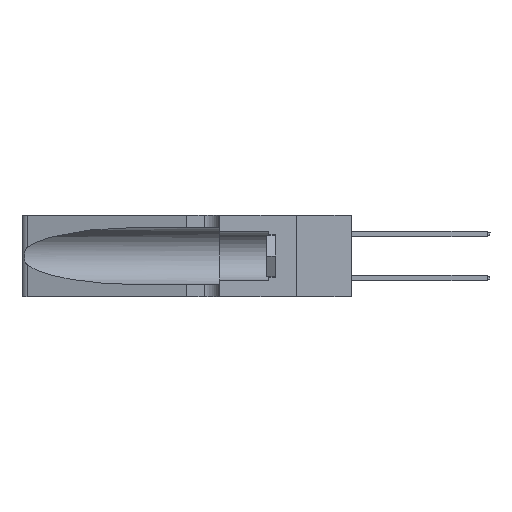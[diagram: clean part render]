
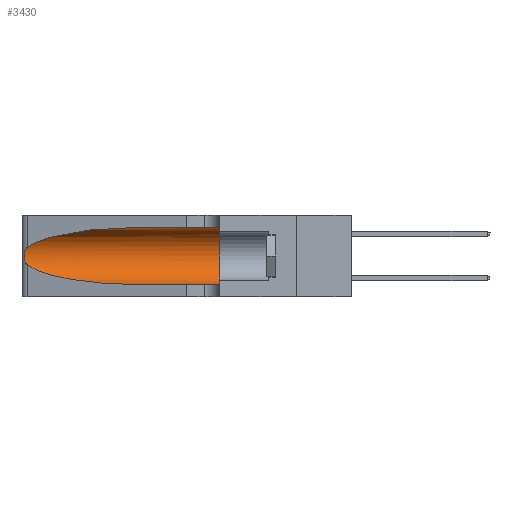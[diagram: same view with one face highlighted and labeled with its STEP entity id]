
A CAD part, left-side view. The second image highlights one B-rep face of the part: STEP entity #3430.
In plain terms, the highlighted cylindrical face has radius 3.308 mm (diameter 6.617 mm), a partial arc.
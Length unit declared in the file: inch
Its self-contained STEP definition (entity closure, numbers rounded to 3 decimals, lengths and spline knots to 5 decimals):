
#22 = CARTESIAN_POINT ( 'NONE',  ( 0.25787, 1.23484, 0.2124 ) ) ;
#74 = VERTEX_POINT ( 'NONE', #20596 ) ;
#368 = EDGE_CURVE ( 'NONE', #74, #1380, #23185, .T. ) ;
#1285 = EDGE_LOOP ( 'NONE', ( #22633, #23891, #3898, #1963, #16253, #22356 ) ) ;
#1380 = VERTEX_POINT ( 'NONE', #8725 ) ;
#1588 = DIRECTION ( 'NONE',  ( 0., 0., 1. ) ) ;
#1607 = DIRECTION ( 'NONE',  ( 0., 1., 0. ) ) ;
#1890 = CARTESIAN_POINT ( 'NONE',  ( 0.18966, 0.96281, 0.05475 ) ) ;
#1963 = ORIENTED_EDGE ( 'NONE', *, *, #10885, .T. ) ;
#2140 = CARTESIAN_POINT ( 'NONE',  ( 0.26018, 1.23835, 0.19895 ) ) ;
#2149 =( BOUNDED_CURVE ( )  B_SPLINE_CURVE ( 3, ( #22498, #5990, #1890, #3976 ),
 .UNSPECIFIED., .F., .F. ) 
 B_SPLINE_CURVE_WITH_KNOTS ( ( 4, 4 ),
 ( 3.44316, 4.71239 ),
 .UNSPECIFIED. ) 
 CURVE ( )  GEOMETRIC_REPRESENTATION_ITEM ( )  RATIONAL_B_SPLINE_CURVE ( ( 1., 0.87, 0.87, 1. ) ) 
 REPRESENTATION_ITEM ( '' )  );
#3423 = EDGE_CURVE ( 'NONE', #4844, #74, #21152, .T. ) ;
#3430 = ADVANCED_FACE ( 'NONE', ( #10179 ), #9531, .F. ) ;
#3793 = EDGE_CURVE ( 'NONE', #21051, #15026, #2149, .T. ) ;
#3898 = ORIENTED_EDGE ( 'NONE', *, *, #3793, .T. ) ;
#3976 = CARTESIAN_POINT ( 'NONE',  ( 0.1305, 0.72297, 0.05475 ) ) ;
#4224 = CARTESIAN_POINT ( 'NONE',  ( 0.26075, 1.23896, 0.178 ) ) ;
#4547 = CARTESIAN_POINT ( 'NONE',  ( 0.1305, 0.72297, 0.05475 ) ) ;
#4634 = VECTOR ( 'NONE', #9175, 39.37008 ) ;
#4844 = VERTEX_POINT ( 'NONE', #26391 ) ;
#4977 =( BOUNDED_CURVE ( )  B_SPLINE_CURVE ( 3, ( #12209, #24491, #26513, #14304 ),
 .UNSPECIFIED., .F., .F. ) 
 B_SPLINE_CURVE_WITH_KNOTS ( ( 4, 4 ),
 ( 1.5708, 2.84003 ),
 .UNSPECIFIED. ) 
 CURVE ( )  GEOMETRIC_REPRESENTATION_ITEM ( )  RATIONAL_B_SPLINE_CURVE ( ( 1., 0.87, 0.87, 1. ) ) 
 REPRESENTATION_ITEM ( '' )  );
#5990 = CARTESIAN_POINT ( 'NONE',  ( 0.2373, 1.15595, 0.08982 ) ) ;
#6043 = VERTEX_POINT ( 'NONE', #21847 ) ;
#6317 = CARTESIAN_POINT ( 'NONE',  ( 0.25856, 1.23593, 0.16098 ) ) ;
#6908 = DIRECTION ( 'NONE',  ( 0., 0., -1. ) ) ;
#7096 = CARTESIAN_POINT ( 'NONE',  ( 0.1305, 1.61858, 0.31525 ) ) ;
#7215 = CARTESIAN_POINT ( 'NONE',  ( 0.1305, 1.61858, 0.05475 ) ) ;
#8436 = CARTESIAN_POINT ( 'NONE',  ( 0.25639, 1.23186, 0.15144 ) ) ;
#8725 = CARTESIAN_POINT ( 'NONE',  ( 0.1305, 0.35, 0.05475 ) ) ;
#9175 = DIRECTION ( 'NONE',  ( 0., -1., 0. ) ) ;
#9531 = CYLINDRICAL_SURFACE ( 'NONE', #14439, 0.13025 ) ;
#10179 = FACE_OUTER_BOUND ( 'NONE', #1285, .T. ) ;
#10399 = CARTESIAN_POINT ( 'NONE',  ( 0.25487, 1.22718, 0.22369 ) ) ;
#10487 = CARTESIAN_POINT ( 'NONE',  ( 0.25487, 1.22718, 0.14631 ) ) ;
#10885 = EDGE_CURVE ( 'NONE', #15026, #1380, #25282, .T. ) ;
#11244 = DIRECTION ( 'NONE',  ( 0., -1., 0. ) ) ;
#11667 = VECTOR ( 'NONE', #21637, 39.37008 ) ;
#12209 = CARTESIAN_POINT ( 'NONE',  ( 0.1305, 0.72297, 0.31525 ) ) ;
#12482 = EDGE_CURVE ( 'NONE', #4844, #6043, #4977, .T. ) ;
#12484 = CARTESIAN_POINT ( 'NONE',  ( 0.25639, 1.23184, 0.21858 ) ) ;
#12627 = B_SPLINE_CURVE_WITH_KNOTS ( 'NONE', 3,
 ( #10399, #20702, #12484, #22, #14586, #2140, #16649, #4224, #18712, #6317, #20793, #8436, #22832, #10487 ),
 .UNSPECIFIED., .F., .F.,
 ( 4, 2, 2, 2, 2, 2, 4 ),
 ( 0., 0.00027, 0.00053, 0.00107, 0.0016, 0.00187, 0.00214 ),
 .UNSPECIFIED. ) ;
#13528 = AXIS2_PLACEMENT_3D ( 'NONE', #19779, #1607, #1588 ) ;
#14304 = CARTESIAN_POINT ( 'NONE',  ( 0.25487, 1.22718, 0.22369 ) ) ;
#14439 = AXIS2_PLACEMENT_3D ( 'NONE', #15333, #11244, #6908 ) ;
#14586 = CARTESIAN_POINT ( 'NONE',  ( 0.25854, 1.2359, 0.20912 ) ) ;
#15026 = VERTEX_POINT ( 'NONE', #4547 ) ;
#15333 = CARTESIAN_POINT ( 'NONE',  ( 0.1305, 1.61858, 0.185 ) ) ;
#16253 = ORIENTED_EDGE ( 'NONE', *, *, #368, .F. ) ;
#16649 = CARTESIAN_POINT ( 'NONE',  ( 0.26075, 1.23896, 0.19203 ) ) ;
#16957 = EDGE_CURVE ( 'NONE', #6043, #21051, #12627, .T. ) ;
#18712 = CARTESIAN_POINT ( 'NONE',  ( 0.26017, 1.23833, 0.17102 ) ) ;
#19779 = CARTESIAN_POINT ( 'NONE',  ( 0.1305, 0.35, 0.185 ) ) ;
#20596 = CARTESIAN_POINT ( 'NONE',  ( 0.1305, 0.35, 0.31525 ) ) ;
#20702 = CARTESIAN_POINT ( 'NONE',  ( 0.25555, 1.22994, 0.2215 ) ) ;
#20793 = CARTESIAN_POINT ( 'NONE',  ( 0.25789, 1.23486, 0.15765 ) ) ;
#21051 = VERTEX_POINT ( 'NONE', #26183 ) ;
#21152 = LINE ( 'NONE', #7096, #4634 ) ;
#21637 = DIRECTION ( 'NONE',  ( 0., -1., 0. ) ) ;
#21847 = CARTESIAN_POINT ( 'NONE',  ( 0.25487, 1.22718, 0.22369 ) ) ;
#22356 = ORIENTED_EDGE ( 'NONE', *, *, #3423, .F. ) ;
#22498 = CARTESIAN_POINT ( 'NONE',  ( 0.25487, 1.22718, 0.14631 ) ) ;
#22633 = ORIENTED_EDGE ( 'NONE', *, *, #12482, .T. ) ;
#22832 = CARTESIAN_POINT ( 'NONE',  ( 0.25555, 1.22993, 0.14849 ) ) ;
#23185 = CIRCLE ( 'NONE', #13528, 0.13025 ) ;
#23891 = ORIENTED_EDGE ( 'NONE', *, *, #16957, .T. ) ;
#24491 = CARTESIAN_POINT ( 'NONE',  ( 0.18966, 0.96281, 0.31525 ) ) ;
#25282 = LINE ( 'NONE', #7215, #11667 ) ;
#26183 = CARTESIAN_POINT ( 'NONE',  ( 0.25487, 1.22718, 0.14631 ) ) ;
#26391 = CARTESIAN_POINT ( 'NONE',  ( 0.1305, 0.72297, 0.31525 ) ) ;
#26513 = CARTESIAN_POINT ( 'NONE',  ( 0.2373, 1.15595, 0.28018 ) ) ;
